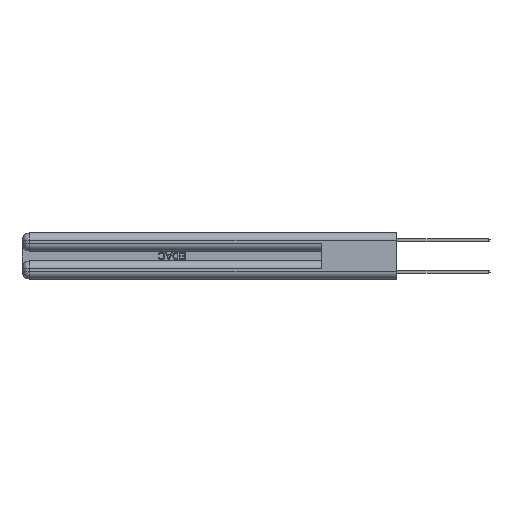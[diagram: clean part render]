
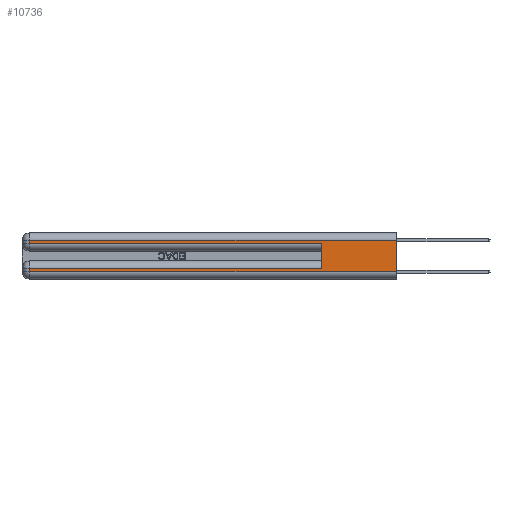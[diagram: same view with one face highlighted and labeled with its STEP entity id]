
A CAD part, left-side view. The second image highlights one B-rep face of the part: STEP entity #10736.
In plain terms, the highlighted planar face has unit normal (-1, 0, 0).
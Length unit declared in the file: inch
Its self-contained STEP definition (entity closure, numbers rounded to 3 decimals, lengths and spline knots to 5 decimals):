
#39 = VERTEX_POINT ( 'NONE', #21137 ) ;
#337 = EDGE_CURVE ( 'NONE', #20787, #22703, #25596, .T. ) ;
#809 = CARTESIAN_POINT ( 'NONE',  ( 0., 2.94, 0.37 ) ) ;
#873 = VERTEX_POINT ( 'NONE', #10710 ) ;
#1512 = CARTESIAN_POINT ( 'NONE',  ( 0., 0.6, 0.145 ) ) ;
#2026 = VECTOR ( 'NONE', #16362, 39.37008 ) ;
#2214 = DIRECTION ( 'NONE',  ( 0., 1., 0. ) ) ;
#2250 = DIRECTION ( 'NONE',  ( 0., 0., -1. ) ) ;
#3889 = VECTOR ( 'NONE', #27750, 39.37008 ) ;
#4206 = CARTESIAN_POINT ( 'NONE',  ( 0., 0., 0.31 ) ) ;
#4286 = LINE ( 'NONE', #1512, #3889 ) ;
#5356 = ORIENTED_EDGE ( 'NONE', *, *, #25454, .T. ) ;
#7415 = ORIENTED_EDGE ( 'NONE', *, *, #25329, .T. ) ;
#7432 = CARTESIAN_POINT ( 'NONE',  ( 0., 0., 0.37 ) ) ;
#8781 = CARTESIAN_POINT ( 'NONE',  ( 0., 0., 0.37 ) ) ;
#9406 = CARTESIAN_POINT ( 'NONE',  ( 0., 2.94, 0.31 ) ) ;
#9877 = EDGE_CURVE ( 'NONE', #39, #873, #4286, .T. ) ;
#10167 = VERTEX_POINT ( 'NONE', #27036 ) ;
#10321 = LINE ( 'NONE', #33807, #18071 ) ;
#10710 = CARTESIAN_POINT ( 'NONE',  ( 0., 0.6, 0.285 ) ) ;
#10736 = ADVANCED_FACE ( 'NONE', ( #25887 ), #33847, .F. ) ;
#10879 = DIRECTION ( 'NONE',  ( 0., 0., -1. ) ) ;
#12321 = DIRECTION ( 'NONE',  ( 0., 1., 0. ) ) ;
#13550 = VERTEX_POINT ( 'NONE', #28292 ) ;
#13928 = CARTESIAN_POINT ( 'NONE',  ( 0., 2.94, 0.085 ) ) ;
#14154 = DIRECTION ( 'NONE',  ( 0., -1., 0. ) ) ;
#15433 = VERTEX_POINT ( 'NONE', #13928 ) ;
#16362 = DIRECTION ( 'NONE',  ( 0., 0., -1. ) ) ;
#16579 = LINE ( 'NONE', #27086, #33748 ) ;
#16703 = LINE ( 'NONE', #809, #31800 ) ;
#17326 = ORIENTED_EDGE ( 'NONE', *, *, #27884, .T. ) ;
#18071 = VECTOR ( 'NONE', #2214, 39.37008 ) ;
#18156 = DIRECTION ( 'NONE',  ( 0., -1., 0. ) ) ;
#20358 = EDGE_LOOP ( 'NONE', ( #22078, #23454, #5356, #30917, #22468, #31959, #7415, #17326 ) ) ;
#20736 = CARTESIAN_POINT ( 'NONE',  ( 0., 0., 0.06 ) ) ;
#20787 = VERTEX_POINT ( 'NONE', #28633 ) ;
#21137 = CARTESIAN_POINT ( 'NONE',  ( 0., 0.6, 0.085 ) ) ;
#21548 = AXIS2_PLACEMENT_3D ( 'NONE', #7432, #30918, #2250 ) ;
#21881 = LINE ( 'NONE', #8781, #32939 ) ;
#22078 = ORIENTED_EDGE ( 'NONE', *, *, #28778, .F. ) ;
#22363 = CARTESIAN_POINT ( 'NONE',  ( 0., 2.94, 0.37 ) ) ;
#22468 = ORIENTED_EDGE ( 'NONE', *, *, #9877, .F. ) ;
#22703 = VERTEX_POINT ( 'NONE', #9406 ) ;
#23425 = VECTOR ( 'NONE', #12321, 39.37008 ) ;
#23454 = ORIENTED_EDGE ( 'NONE', *, *, #337, .T. ) ;
#25329 = EDGE_CURVE ( 'NONE', #15433, #10167, #16703, .T. ) ;
#25454 = EDGE_CURVE ( 'NONE', #22703, #29842, #27377, .T. ) ;
#25596 = LINE ( 'NONE', #4206, #23425 ) ;
#25887 = FACE_OUTER_BOUND ( 'NONE', #20358, .T. ) ;
#26065 = LINE ( 'NONE', #20736, #31323 ) ;
#27036 = CARTESIAN_POINT ( 'NONE',  ( 0., 2.94, 0.06 ) ) ;
#27086 = CARTESIAN_POINT ( 'NONE',  ( 0., 0., 0.285 ) ) ;
#27377 = LINE ( 'NONE', #22363, #2026 ) ;
#27750 = DIRECTION ( 'NONE',  ( 0., 0., 1. ) ) ;
#27884 = EDGE_CURVE ( 'NONE', #10167, #13550, #26065, .T. ) ;
#28292 = CARTESIAN_POINT ( 'NONE',  ( 0., 0., 0.06 ) ) ;
#28633 = CARTESIAN_POINT ( 'NONE',  ( 0., 0., 0.31 ) ) ;
#28716 = CARTESIAN_POINT ( 'NONE',  ( 0., 2.94, 0.285 ) ) ;
#28778 = EDGE_CURVE ( 'NONE', #20787, #13550, #21881, .T. ) ;
#29013 = EDGE_CURVE ( 'NONE', #39, #15433, #10321, .T. ) ;
#29842 = VERTEX_POINT ( 'NONE', #28716 ) ;
#29984 = DIRECTION ( 'NONE',  ( 0., 0., -1. ) ) ;
#30917 = ORIENTED_EDGE ( 'NONE', *, *, #33970, .T. ) ;
#30918 = DIRECTION ( 'NONE',  ( 1., 0., 0. ) ) ;
#31323 = VECTOR ( 'NONE', #18156, 39.37008 ) ;
#31800 = VECTOR ( 'NONE', #29984, 39.37008 ) ;
#31959 = ORIENTED_EDGE ( 'NONE', *, *, #29013, .T. ) ;
#32939 = VECTOR ( 'NONE', #10879, 39.37008 ) ;
#33748 = VECTOR ( 'NONE', #14154, 39.37008 ) ;
#33807 = CARTESIAN_POINT ( 'NONE',  ( 0., 0., 0.085 ) ) ;
#33847 = PLANE ( 'NONE',  #21548 ) ;
#33970 = EDGE_CURVE ( 'NONE', #29842, #873, #16579, .T. ) ;
